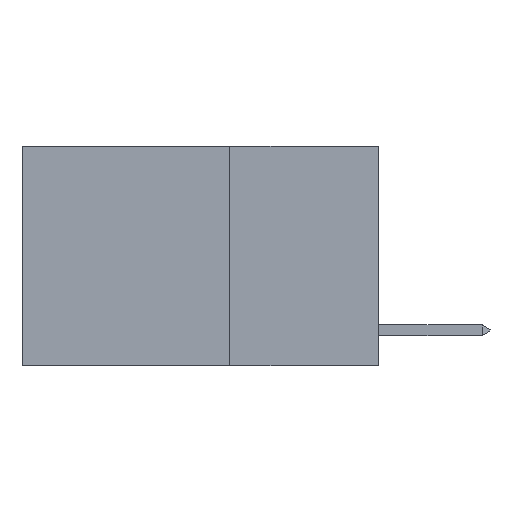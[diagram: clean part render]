
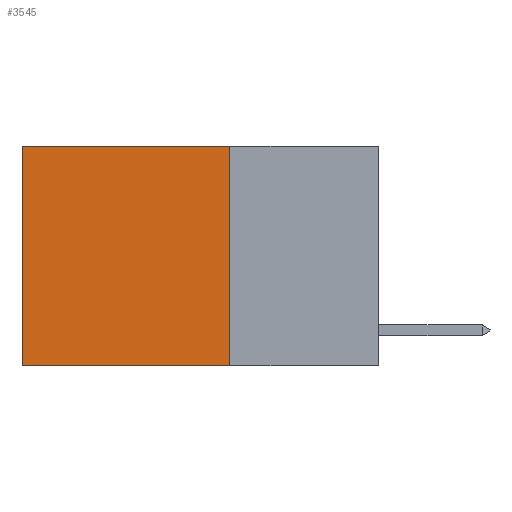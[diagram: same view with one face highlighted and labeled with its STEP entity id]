
A CAD part, left-side view. The second image highlights one B-rep face of the part: STEP entity #3545.
In plain terms, the highlighted planar face has unit normal (-1, 0, 0).
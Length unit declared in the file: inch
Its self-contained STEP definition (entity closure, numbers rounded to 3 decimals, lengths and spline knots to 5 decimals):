
#55 = ORIENTED_EDGE ( 'NONE', *, *, #5770, .T. ) ;
#1250 = CARTESIAN_POINT ( 'NONE',  ( 0.2625, 0.6, -0.37 ) ) ;
#1433 = LINE ( 'NONE', #16449, #12445 ) ;
#1993 = DIRECTION ( 'NONE',  ( 0., 0., -1. ) ) ;
#2519 = VECTOR ( 'NONE', #1993, 39.37008 ) ;
#3434 = CARTESIAN_POINT ( 'NONE',  ( 0.2625, 0.25, 0. ) ) ;
#3545 = ADVANCED_FACE ( 'NONE', ( #16858 ), #12016, .F. ) ;
#4601 = EDGE_CURVE ( 'NONE', #9799, #17742, #10498, .T. ) ;
#4867 = DIRECTION ( 'NONE',  ( 1., 0., 0. ) ) ;
#5070 = ORIENTED_EDGE ( 'NONE', *, *, #4601, .F. ) ;
#5074 = VECTOR ( 'NONE', #11100, 39.37008 ) ;
#5175 = VERTEX_POINT ( 'NONE', #15514 ) ;
#5770 = EDGE_CURVE ( 'NONE', #17861, #17742, #8897, .T. ) ;
#6375 = LINE ( 'NONE', #10576, #2519 ) ;
#6804 = CARTESIAN_POINT ( 'NONE',  ( 0.2625, 0.6, 0. ) ) ;
#7090 = CARTESIAN_POINT ( 'NONE',  ( 0.2625, 0.25, -0.37 ) ) ;
#7447 = CARTESIAN_POINT ( 'NONE',  ( 0.2625, 0.25, -0.37 ) ) ;
#7479 = EDGE_CURVE ( 'NONE', #5175, #9799, #6375, .T. ) ;
#7813 = DIRECTION ( 'NONE',  ( 0., 1., 0. ) ) ;
#8897 = LINE ( 'NONE', #6804, #5074 ) ;
#9799 = VERTEX_POINT ( 'NONE', #7447 ) ;
#10225 = ORIENTED_EDGE ( 'NONE', *, *, #7479, .F. ) ;
#10498 = LINE ( 'NONE', #7090, #15278 ) ;
#10576 = CARTESIAN_POINT ( 'NONE',  ( 0.2625, 0.25, 0. ) ) ;
#11100 = DIRECTION ( 'NONE',  ( 0., 0., -1. ) ) ;
#12016 = PLANE ( 'NONE',  #13409 ) ;
#12445 = VECTOR ( 'NONE', #7813, 39.37008 ) ;
#13006 = CARTESIAN_POINT ( 'NONE',  ( 0.2625, 0.6, 0. ) ) ;
#13409 = AXIS2_PLACEMENT_3D ( 'NONE', #3434, #4867, #14956 ) ;
#14070 = ORIENTED_EDGE ( 'NONE', *, *, #14267, .T. ) ;
#14257 = DIRECTION ( 'NONE',  ( 0., 1., 0. ) ) ;
#14267 = EDGE_CURVE ( 'NONE', #5175, #17861, #1433, .T. ) ;
#14682 = EDGE_LOOP ( 'NONE', ( #55, #5070, #10225, #14070 ) ) ;
#14956 = DIRECTION ( 'NONE',  ( 0., 0., -1. ) ) ;
#15278 = VECTOR ( 'NONE', #14257, 39.37008 ) ;
#15514 = CARTESIAN_POINT ( 'NONE',  ( 0.2625, 0.25, 0. ) ) ;
#16449 = CARTESIAN_POINT ( 'NONE',  ( 0.2625, 0.25, 0. ) ) ;
#16858 = FACE_OUTER_BOUND ( 'NONE', #14682, .T. ) ;
#17742 = VERTEX_POINT ( 'NONE', #1250 ) ;
#17861 = VERTEX_POINT ( 'NONE', #13006 ) ;
